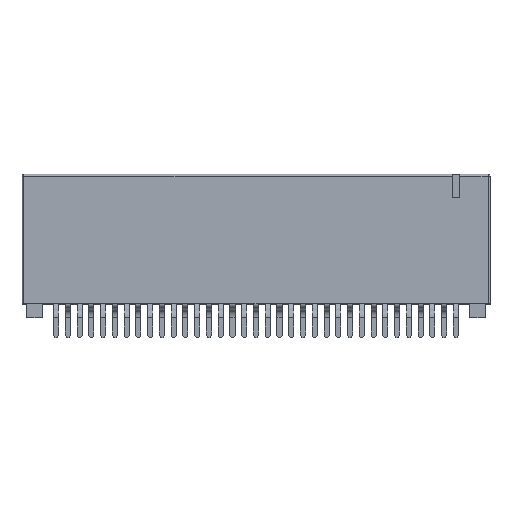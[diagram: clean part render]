
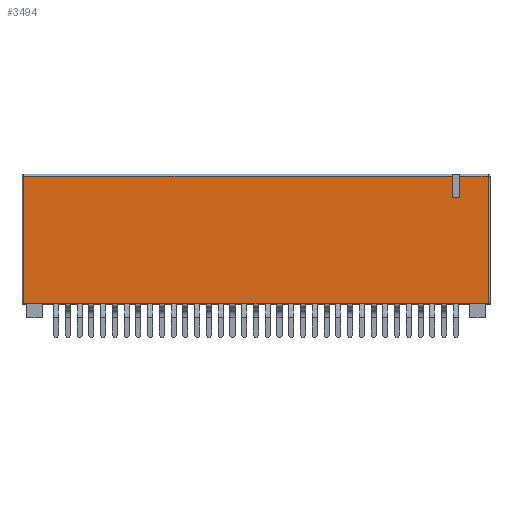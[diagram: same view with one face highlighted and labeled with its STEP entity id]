
A CAD part, top view. The second image highlights one B-rep face of the part: STEP entity #3494.
In plain terms, the highlighted planar face has unit normal (0, 0, 1).
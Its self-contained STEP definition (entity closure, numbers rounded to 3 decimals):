
#12 = DIRECTION ( 'NONE',  ( -1., 0., 0. ) ) ;
#43 = VERTEX_POINT ( 'NONE', #8144 ) ;
#432 = LINE ( 'NONE', #7450, #15901 ) ;
#2149 = CARTESIAN_POINT ( 'NONE',  ( 46.475, 15.3, 0. ) ) ;
#2373 = EDGE_CURVE ( 'NONE', #17654, #11180, #7179, .T. ) ;
#3494 = ADVANCED_FACE ( 'NONE', ( #4982 ), #25326, .F. ) ;
#4042 = EDGE_CURVE ( 'NONE', #43, #23468, #22021, .T. ) ;
#4093 = LINE ( 'NONE', #10972, #7028 ) ;
#4421 = AXIS2_PLACEMENT_3D ( 'NONE', #21079, #5554, #5414 ) ;
#4711 = EDGE_CURVE ( 'NONE', #25067, #28245, #28843, .T. ) ;
#4889 = VECTOR ( 'NONE', #12, 1000. ) ;
#4982 = FACE_OUTER_BOUND ( 'NONE', #11208, .T. ) ;
#5414 = DIRECTION ( 'NONE',  ( -1., 0., 0. ) ) ;
#5540 = CARTESIAN_POINT ( 'NONE',  ( 50.35, 1.5, 0. ) ) ;
#5554 = DIRECTION ( 'NONE',  ( 0., 0., -1. ) ) ;
#5864 = VECTOR ( 'NONE', #21591, 1000. ) ;
#6358 = CARTESIAN_POINT ( 'NONE',  ( 46.475, 12.95, 0. ) ) ;
#6475 = DIRECTION ( 'NONE',  ( 0., 1., 0. ) ) ;
#7028 = VECTOR ( 'NONE', #28824, 1000. ) ;
#7179 = LINE ( 'NONE', #27240, #24267 ) ;
#7450 = CARTESIAN_POINT ( 'NONE',  ( 47.255, 12.95, 0. ) ) ;
#7753 = DIRECTION ( 'NONE',  ( -1., 0., 0. ) ) ;
#8065 = DIRECTION ( 'NONE',  ( 0., -1., 0. ) ) ;
#8127 = CARTESIAN_POINT ( 'NONE',  ( 46.475, 12.95, 0. ) ) ;
#8144 = CARTESIAN_POINT ( 'NONE',  ( 46.475, 12.95, 0. ) ) ;
#8240 = LINE ( 'NONE', #19512, #12634 ) ;
#8273 = ORIENTED_EDGE ( 'NONE', *, *, #4711, .T. ) ;
#10972 = CARTESIAN_POINT ( 'NONE',  ( 50.35, 15.5, 0. ) ) ;
#11180 = VERTEX_POINT ( 'NONE', #23301 ) ;
#11208 = EDGE_LOOP ( 'NONE', ( #23142, #14526, #23019, #26943, #27712, #25573, #8273, #25608 ) ) ;
#11342 = CARTESIAN_POINT ( 'NONE',  ( 50.35, 15.3, 0. ) ) ;
#12634 = VECTOR ( 'NONE', #23760, 1000. ) ;
#13428 = EDGE_CURVE ( 'NONE', #43, #14350, #28176, .T. ) ;
#13971 = CARTESIAN_POINT ( 'NONE',  ( 47.255, 12.95, 0. ) ) ;
#14350 = VERTEX_POINT ( 'NONE', #2149 ) ;
#14526 = ORIENTED_EDGE ( 'NONE', *, *, #13428, .T. ) ;
#15901 = VECTOR ( 'NONE', #6475, 1000. ) ;
#17051 = DIRECTION ( 'NONE',  ( 0., 1., 0. ) ) ;
#17307 = EDGE_CURVE ( 'NONE', #17654, #25067, #4093, .T. ) ;
#17654 = VERTEX_POINT ( 'NONE', #5540 ) ;
#18502 = EDGE_CURVE ( 'NONE', #26332, #11180, #28111, .T. ) ;
#19512 = CARTESIAN_POINT ( 'NONE',  ( 0., 15.3, 0. ) ) ;
#21079 = CARTESIAN_POINT ( 'NONE',  ( 0., 15.5, 0. ) ) ;
#21591 = DIRECTION ( 'NONE',  ( 1., 0., 0. ) ) ;
#22021 = LINE ( 'NONE', #6358, #5864 ) ;
#22472 = CARTESIAN_POINT ( 'NONE',  ( 0.2, 15.3, 0. ) ) ;
#22712 = CARTESIAN_POINT ( 'NONE',  ( 0., 15.3, 0. ) ) ;
#22802 = VECTOR ( 'NONE', #8065, 1000. ) ;
#23019 = ORIENTED_EDGE ( 'NONE', *, *, #25297, .T. ) ;
#23142 = ORIENTED_EDGE ( 'NONE', *, *, #4042, .F. ) ;
#23163 = CARTESIAN_POINT ( 'NONE',  ( 47.255, 15.3, 0. ) ) ;
#23301 = CARTESIAN_POINT ( 'NONE',  ( 0.2, 1.5, 0. ) ) ;
#23468 = VERTEX_POINT ( 'NONE', #13971 ) ;
#23583 = CARTESIAN_POINT ( 'NONE',  ( 0.2, 15.5, 0. ) ) ;
#23760 = DIRECTION ( 'NONE',  ( -1., 0., 0. ) ) ;
#24267 = VECTOR ( 'NONE', #7753, 1000. ) ;
#25067 = VERTEX_POINT ( 'NONE', #11342 ) ;
#25297 = EDGE_CURVE ( 'NONE', #14350, #26332, #8240, .T. ) ;
#25326 = PLANE ( 'NONE',  #4421 ) ;
#25436 = EDGE_CURVE ( 'NONE', #23468, #28245, #432, .T. ) ;
#25520 = VECTOR ( 'NONE', #17051, 1000. ) ;
#25573 = ORIENTED_EDGE ( 'NONE', *, *, #17307, .T. ) ;
#25608 = ORIENTED_EDGE ( 'NONE', *, *, #25436, .F. ) ;
#26332 = VERTEX_POINT ( 'NONE', #22472 ) ;
#26943 = ORIENTED_EDGE ( 'NONE', *, *, #18502, .T. ) ;
#27240 = CARTESIAN_POINT ( 'NONE',  ( 50.55, 1.5, 0. ) ) ;
#27712 = ORIENTED_EDGE ( 'NONE', *, *, #2373, .F. ) ;
#28111 = LINE ( 'NONE', #23583, #22802 ) ;
#28176 = LINE ( 'NONE', #8127, #25520 ) ;
#28245 = VERTEX_POINT ( 'NONE', #23163 ) ;
#28824 = DIRECTION ( 'NONE',  ( 0., 1., 0. ) ) ;
#28843 = LINE ( 'NONE', #22712, #4889 ) ;
